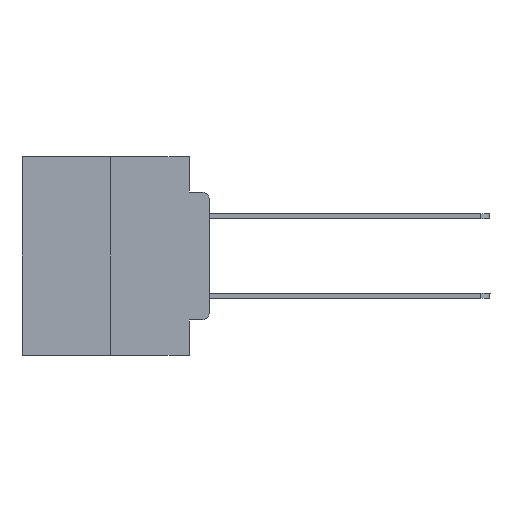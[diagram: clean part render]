
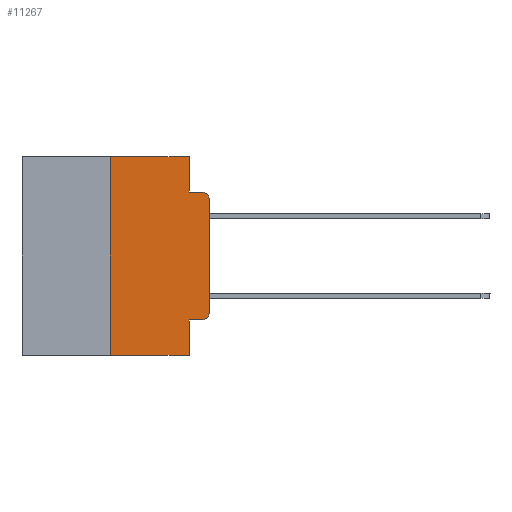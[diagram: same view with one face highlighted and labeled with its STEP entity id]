
A CAD part, left-side view. The second image highlights one B-rep face of the part: STEP entity #11267.
In plain terms, the highlighted planar face has unit normal (-1, 0, 0).
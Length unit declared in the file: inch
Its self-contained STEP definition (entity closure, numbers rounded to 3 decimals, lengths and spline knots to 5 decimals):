
#302 = EDGE_CURVE ( 'NONE', #24907, #20187, #19635, .T. ) ;
#670 = DIRECTION ( 'NONE',  ( 0., -1., 0. ) ) ;
#1599 = VECTOR ( 'NONE', #6458, 39.37008 ) ;
#1822 = LINE ( 'NONE', #23817, #1599 ) ;
#2380 = VECTOR ( 'NONE', #2467, 39.37008 ) ;
#2444 = VERTEX_POINT ( 'NONE', #4190 ) ;
#2451 = CIRCLE ( 'NONE', #23695, 0.02 ) ;
#2467 = DIRECTION ( 'NONE',  ( 0., 0., -1. ) ) ;
#2757 = LINE ( 'NONE', #27052, #13321 ) ;
#2959 = DIRECTION ( 'NONE',  ( 0., 0., -1. ) ) ;
#3824 = VERTEX_POINT ( 'NONE', #11355 ) ;
#4148 = VERTEX_POINT ( 'NONE', #6254 ) ;
#4190 = CARTESIAN_POINT ( 'NONE',  ( 0., 0., -0.3915 ) ) ;
#5562 = VERTEX_POINT ( 'NONE', #6837 ) ;
#6177 = ORIENTED_EDGE ( 'NONE', *, *, #23551, .T. ) ;
#6181 = EDGE_CURVE ( 'NONE', #2444, #24907, #2757, .T. ) ;
#6254 = CARTESIAN_POINT ( 'NONE',  ( 0., 0.051, -0.4115 ) ) ;
#6394 = DIRECTION ( 'NONE',  ( 1., 0., 0. ) ) ;
#6458 = DIRECTION ( 'NONE',  ( 0., -1., 0. ) ) ;
#6837 = CARTESIAN_POINT ( 'NONE',  ( 0., 0.051, 0. ) ) ;
#7031 = VECTOR ( 'NONE', #24031, 39.37008 ) ;
#8576 = DIRECTION ( 'NONE',  ( -1., 0., 0. ) ) ;
#8671 = ORIENTED_EDGE ( 'NONE', *, *, #12581, .F. ) ;
#8741 = CARTESIAN_POINT ( 'NONE',  ( 0., 0.02, -0.0885 ) ) ;
#9448 = ORIENTED_EDGE ( 'NONE', *, *, #26057, .T. ) ;
#9460 = CARTESIAN_POINT ( 'NONE',  ( 0., 0.02, -0.1085 ) ) ;
#10172 = AXIS2_PLACEMENT_3D ( 'NONE', #19027, #6394, #15231 ) ;
#10523 = VECTOR ( 'NONE', #17078, 39.37008 ) ;
#11016 = EDGE_CURVE ( 'NONE', #28006, #5562, #27419, .T. ) ;
#11267 = ADVANCED_FACE ( 'NONE', ( #26220 ), #16694, .F. ) ;
#11355 = CARTESIAN_POINT ( 'NONE',  ( 0., 0.051, -0.0885 ) ) ;
#12581 = EDGE_CURVE ( 'NONE', #5562, #3824, #28500, .T. ) ;
#12588 = VECTOR ( 'NONE', #15743, 39.37008 ) ;
#13024 = CARTESIAN_POINT ( 'NONE',  ( 0., 0.051, 0. ) ) ;
#13029 = CARTESIAN_POINT ( 'NONE',  ( 0., 0.473, -0.5 ) ) ;
#13321 = VECTOR ( 'NONE', #23132, 39.37008 ) ;
#13458 = DIRECTION ( 'NONE',  ( 0., 0., -1. ) ) ;
#13888 = CARTESIAN_POINT ( 'NONE',  ( 0., 0.051, 0. ) ) ;
#14773 = VECTOR ( 'NONE', #670, 39.37008 ) ;
#15231 = DIRECTION ( 'NONE',  ( 0., 0., -1. ) ) ;
#15282 = CARTESIAN_POINT ( 'NONE',  ( 0., 0.051, -0.5 ) ) ;
#15305 = ORIENTED_EDGE ( 'NONE', *, *, #11016, .F. ) ;
#15503 = LINE ( 'NONE', #13888, #15921 ) ;
#15743 = DIRECTION ( 'NONE',  ( 0., 0., 1. ) ) ;
#15765 = ORIENTED_EDGE ( 'NONE', *, *, #17601, .F. ) ;
#15921 = VECTOR ( 'NONE', #13458, 39.37008 ) ;
#16694 = PLANE ( 'NONE',  #10172 ) ;
#16815 = EDGE_CURVE ( 'NONE', #4148, #21297, #15503, .T. ) ;
#17078 = DIRECTION ( 'NONE',  ( 0., -1., 0. ) ) ;
#17601 = EDGE_CURVE ( 'NONE', #3824, #20187, #1822, .T. ) ;
#17657 = CARTESIAN_POINT ( 'NONE',  ( 0., 0., -0.1085 ) ) ;
#17744 = VERTEX_POINT ( 'NONE', #24674 ) ;
#18105 = LINE ( 'NONE', #13029, #7031 ) ;
#18982 = LINE ( 'NONE', #28071, #10523 ) ;
#19027 = CARTESIAN_POINT ( 'NONE',  ( 0., 0.473, 0. ) ) ;
#19635 = CIRCLE ( 'NONE', #21458, 0.02 ) ;
#20187 = VERTEX_POINT ( 'NONE', #8741 ) ;
#20290 = CARTESIAN_POINT ( 'NONE',  ( 0., 0.25, 0. ) ) ;
#20398 = ORIENTED_EDGE ( 'NONE', *, *, #23750, .F. ) ;
#21019 = ORIENTED_EDGE ( 'NONE', *, *, #22128, .T. ) ;
#21227 = CARTESIAN_POINT ( 'NONE',  ( 0., 0.25, -0.5 ) ) ;
#21297 = VERTEX_POINT ( 'NONE', #15282 ) ;
#21458 = AXIS2_PLACEMENT_3D ( 'NONE', #9460, #23066, #2959 ) ;
#21615 = CARTESIAN_POINT ( 'NONE',  ( 0., 0.02, -0.3915 ) ) ;
#22128 = EDGE_CURVE ( 'NONE', #4148, #17744, #18982, .T. ) ;
#22664 = CARTESIAN_POINT ( 'NONE',  ( 0., 0.473, 0. ) ) ;
#23066 = DIRECTION ( 'NONE',  ( -1., 0., 0. ) ) ;
#23132 = DIRECTION ( 'NONE',  ( 0., 0., 1. ) ) ;
#23551 = EDGE_CURVE ( 'NONE', #26769, #21297, #18105, .T. ) ;
#23695 = AXIS2_PLACEMENT_3D ( 'NONE', #21615, #8576, #23930 ) ;
#23750 = EDGE_CURVE ( 'NONE', #26769, #28006, #26590, .T. ) ;
#23817 = CARTESIAN_POINT ( 'NONE',  ( 0., 0.051, -0.0885 ) ) ;
#23930 = DIRECTION ( 'NONE',  ( 0., 0., -1. ) ) ;
#24031 = DIRECTION ( 'NONE',  ( 0., -1., 0. ) ) ;
#24412 = CARTESIAN_POINT ( 'NONE',  ( 0., 0.25, 0. ) ) ;
#24674 = CARTESIAN_POINT ( 'NONE',  ( 0., 0.02, -0.4115 ) ) ;
#24907 = VERTEX_POINT ( 'NONE', #17657 ) ;
#25589 = ORIENTED_EDGE ( 'NONE', *, *, #302, .T. ) ;
#26057 = EDGE_CURVE ( 'NONE', #17744, #2444, #2451, .T. ) ;
#26220 = FACE_OUTER_BOUND ( 'NONE', #27801, .T. ) ;
#26590 = LINE ( 'NONE', #24412, #12588 ) ;
#26769 = VERTEX_POINT ( 'NONE', #21227 ) ;
#26901 = ORIENTED_EDGE ( 'NONE', *, *, #6181, .T. ) ;
#27052 = CARTESIAN_POINT ( 'NONE',  ( 0., 0., 0. ) ) ;
#27290 = ORIENTED_EDGE ( 'NONE', *, *, #16815, .F. ) ;
#27419 = LINE ( 'NONE', #22664, #14773 ) ;
#27801 = EDGE_LOOP ( 'NONE', ( #26901, #25589, #15765, #8671, #15305, #20398, #6177, #27290, #21019, #9448 ) ) ;
#28006 = VERTEX_POINT ( 'NONE', #20290 ) ;
#28071 = CARTESIAN_POINT ( 'NONE',  ( 0., 0.051, -0.4115 ) ) ;
#28500 = LINE ( 'NONE', #13024, #2380 ) ;
